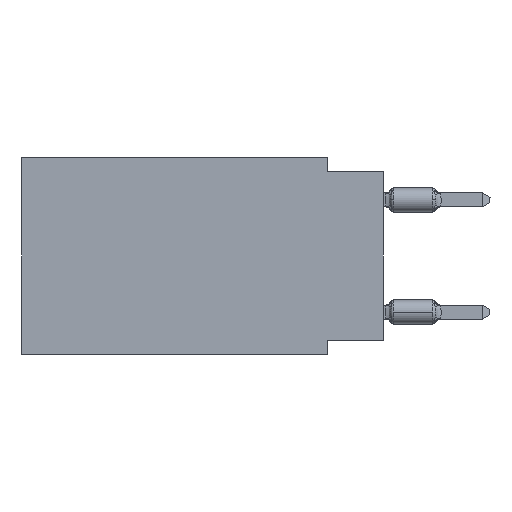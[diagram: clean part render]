
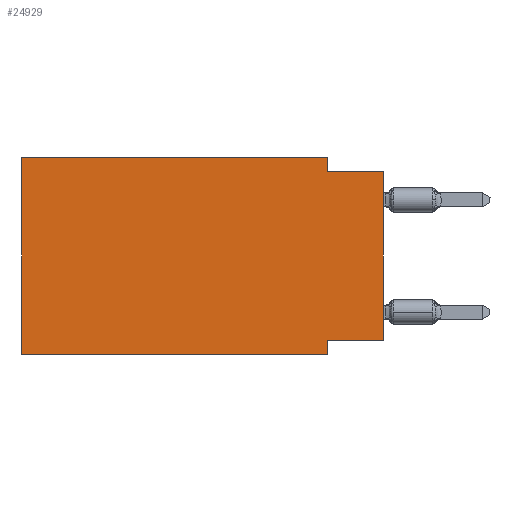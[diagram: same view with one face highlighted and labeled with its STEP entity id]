
A CAD part, left-side view. The second image highlights one B-rep face of the part: STEP entity #24929.
In plain terms, the highlighted planar face has unit normal (-1, 0, 0).
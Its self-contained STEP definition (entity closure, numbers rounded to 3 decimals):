
#208 = CARTESIAN_POINT ( 'NONE',  ( 0., 16.383, 0. ) ) ;
#470 = VERTEX_POINT ( 'NONE', #19343 ) ;
#1069 = DIRECTION ( 'NONE',  ( 0., -1., 0. ) ) ;
#1189 = CARTESIAN_POINT ( 'NONE',  ( 0., 0., -0.635 ) ) ;
#2521 = EDGE_CURVE ( 'NONE', #41953, #41558, #28074, .T. ) ;
#3396 = DIRECTION ( 'NONE',  ( 0., 0., -1. ) ) ;
#3440 = CARTESIAN_POINT ( 'NONE',  ( 0., 0., -8.255 ) ) ;
#5049 = VECTOR ( 'NONE', #30730, 1000. ) ;
#5144 = FACE_OUTER_BOUND ( 'NONE', #34418, .T. ) ;
#5259 = CARTESIAN_POINT ( 'NONE',  ( 0., 16.383, 0. ) ) ;
#5291 = CARTESIAN_POINT ( 'NONE',  ( 0., 0., -8.255 ) ) ;
#5980 = EDGE_CURVE ( 'NONE', #39298, #13183, #22750, .T. ) ;
#6086 = ORIENTED_EDGE ( 'NONE', *, *, #42693, .F. ) ;
#6429 = AXIS2_PLACEMENT_3D ( 'NONE', #23270, #40945, #33747 ) ;
#6545 = VERTEX_POINT ( 'NONE', #27555 ) ;
#8408 = PLANE ( 'NONE',  #6429 ) ;
#9747 = ORIENTED_EDGE ( 'NONE', *, *, #11219, .F. ) ;
#9787 = VECTOR ( 'NONE', #23541, 1000. ) ;
#11219 = EDGE_CURVE ( 'NONE', #6545, #35965, #13687, .T. ) ;
#12410 = ORIENTED_EDGE ( 'NONE', *, *, #2521, .F. ) ;
#12976 = DIRECTION ( 'NONE',  ( 0., 0., 1. ) ) ;
#13183 = VERTEX_POINT ( 'NONE', #22737 ) ;
#13295 = LINE ( 'NONE', #27495, #9787 ) ;
#13511 = EDGE_CURVE ( 'NONE', #6545, #470, #29439, .T. ) ;
#13687 = LINE ( 'NONE', #208, #25404 ) ;
#14298 = VECTOR ( 'NONE', #3396, 1000. ) ;
#15391 = ORIENTED_EDGE ( 'NONE', *, *, #27500, .F. ) ;
#16006 = CARTESIAN_POINT ( 'NONE',  ( 0., 0., 0. ) ) ;
#16537 = CARTESIAN_POINT ( 'NONE',  ( 0., 0., -0.635 ) ) ;
#16978 = EDGE_CURVE ( 'NONE', #13183, #470, #13295, .T. ) ;
#17193 = VERTEX_POINT ( 'NONE', #1189 ) ;
#18075 = VECTOR ( 'NONE', #33637, 1000. ) ;
#19343 = CARTESIAN_POINT ( 'NONE',  ( 0., 2.54, -8.89 ) ) ;
#20886 = DIRECTION ( 'NONE',  ( 0., 0., 1. ) ) ;
#22073 = VECTOR ( 'NONE', #22524, 1000. ) ;
#22248 = ORIENTED_EDGE ( 'NONE', *, *, #34692, .T. ) ;
#22524 = DIRECTION ( 'NONE',  ( 0., 1., 0. ) ) ;
#22737 = CARTESIAN_POINT ( 'NONE',  ( 0., 2.54, -8.255 ) ) ;
#22750 = LINE ( 'NONE', #5291, #22073 ) ;
#23270 = CARTESIAN_POINT ( 'NONE',  ( 0., 16.383, 0. ) ) ;
#23541 = DIRECTION ( 'NONE',  ( 0., 0., -1. ) ) ;
#24185 = ORIENTED_EDGE ( 'NONE', *, *, #5980, .F. ) ;
#24929 = ADVANCED_FACE ( 'NONE', ( #5144 ), #8408, .F. ) ;
#25183 = ORIENTED_EDGE ( 'NONE', *, *, #13511, .T. ) ;
#25404 = VECTOR ( 'NONE', #20886, 1000. ) ;
#25552 = VECTOR ( 'NONE', #12976, 1000. ) ;
#26793 = LINE ( 'NONE', #16537, #5049 ) ;
#27495 = CARTESIAN_POINT ( 'NONE',  ( 0., 2.54, -8.89 ) ) ;
#27500 = EDGE_CURVE ( 'NONE', #41558, #17193, #26793, .T. ) ;
#27555 = CARTESIAN_POINT ( 'NONE',  ( 0., 16.383, -8.89 ) ) ;
#28074 = LINE ( 'NONE', #28291, #14298 ) ;
#28291 = CARTESIAN_POINT ( 'NONE',  ( 0., 2.54, 0. ) ) ;
#29439 = LINE ( 'NONE', #36417, #45634 ) ;
#30730 = DIRECTION ( 'NONE',  ( 0., -1., 0. ) ) ;
#33637 = DIRECTION ( 'NONE',  ( 0., -1., 0. ) ) ;
#33747 = DIRECTION ( 'NONE',  ( 0., 0., -1. ) ) ;
#33795 = CARTESIAN_POINT ( 'NONE',  ( 0., 2.54, 0. ) ) ;
#34418 = EDGE_LOOP ( 'NONE', ( #22248, #15391, #12410, #6086, #9747, #25183, #36280, #24185 ) ) ;
#34692 = EDGE_CURVE ( 'NONE', #39298, #17193, #44836, .T. ) ;
#35965 = VERTEX_POINT ( 'NONE', #44442 ) ;
#36280 = ORIENTED_EDGE ( 'NONE', *, *, #16978, .F. ) ;
#36417 = CARTESIAN_POINT ( 'NONE',  ( 0., 16.383, -8.89 ) ) ;
#37134 = LINE ( 'NONE', #5259, #18075 ) ;
#39298 = VERTEX_POINT ( 'NONE', #3440 ) ;
#40945 = DIRECTION ( 'NONE',  ( 1., 0., 0. ) ) ;
#41558 = VERTEX_POINT ( 'NONE', #45243 ) ;
#41953 = VERTEX_POINT ( 'NONE', #33795 ) ;
#42693 = EDGE_CURVE ( 'NONE', #35965, #41953, #37134, .T. ) ;
#44442 = CARTESIAN_POINT ( 'NONE',  ( 0., 16.383, 0. ) ) ;
#44836 = LINE ( 'NONE', #16006, #25552 ) ;
#45243 = CARTESIAN_POINT ( 'NONE',  ( 0., 2.54, -0.635 ) ) ;
#45634 = VECTOR ( 'NONE', #1069, 1000. ) ;
